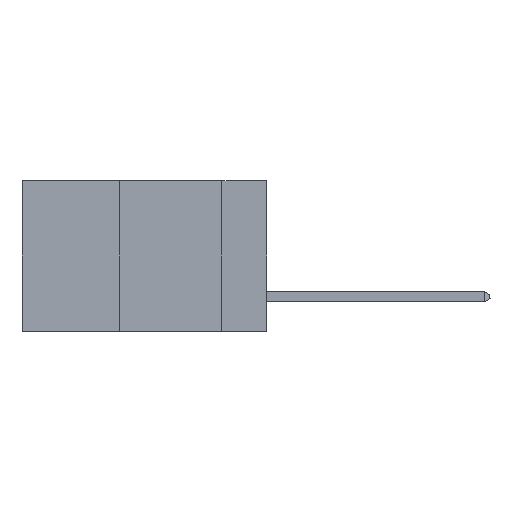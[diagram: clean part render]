
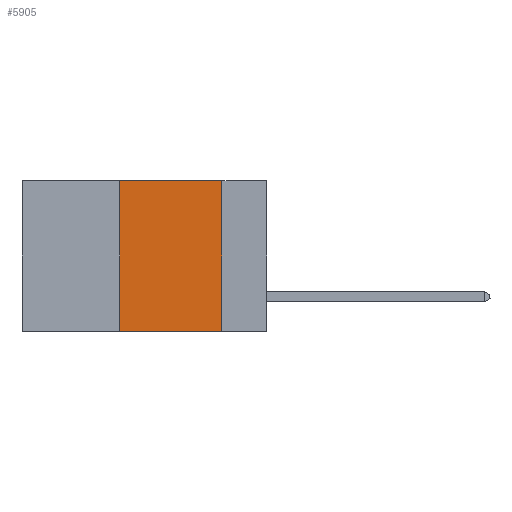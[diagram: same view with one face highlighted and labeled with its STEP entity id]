
A CAD part, left-side view. The second image highlights one B-rep face of the part: STEP entity #5905.
In plain terms, the highlighted planar face has unit normal (-1, 0, 0).
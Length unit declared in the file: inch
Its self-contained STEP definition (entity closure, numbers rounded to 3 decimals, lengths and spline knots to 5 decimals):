
#2057 = DIRECTION ( 'NONE',  ( 0., 0., -1. ) ) ;
#2290 = CARTESIAN_POINT ( 'NONE',  ( 0., 0.36, 0. ) ) ;
#3168 = DIRECTION ( 'NONE',  ( 0., 0., -1. ) ) ;
#3203 = VECTOR ( 'NONE', #41339, 39.37008 ) ;
#4285 = ORIENTED_EDGE ( 'NONE', *, *, #36678, .T. ) ;
#5442 = VERTEX_POINT ( 'NONE', #39004 ) ;
#5522 = LINE ( 'NONE', #34456, #35684 ) ;
#5905 = ADVANCED_FACE ( 'NONE', ( #32025 ), #12707, .F. ) ;
#6354 = LINE ( 'NONE', #30310, #41533 ) ;
#6455 = ORIENTED_EDGE ( 'NONE', *, *, #17333, .F. ) ;
#11524 = LINE ( 'NONE', #25259, #29942 ) ;
#12090 = DIRECTION ( 'NONE',  ( 0., 0., 1. ) ) ;
#12243 = EDGE_LOOP ( 'NONE', ( #38064, #12411, #6455, #4285 ) ) ;
#12411 = ORIENTED_EDGE ( 'NONE', *, *, #16439, .F. ) ;
#12707 = PLANE ( 'NONE',  #27489 ) ;
#15967 = DIRECTION ( 'NONE',  ( 0., -1., 0. ) ) ;
#16439 = EDGE_CURVE ( 'NONE', #20445, #27899, #11524, .T. ) ;
#17333 = EDGE_CURVE ( 'NONE', #5442, #20445, #6354, .T. ) ;
#20445 = VERTEX_POINT ( 'NONE', #2290 ) ;
#25259 = CARTESIAN_POINT ( 'NONE',  ( 0., 0.6, 0. ) ) ;
#25865 = CARTESIAN_POINT ( 'NONE',  ( 0., 0.6, 0. ) ) ;
#27489 = AXIS2_PLACEMENT_3D ( 'NONE', #25865, #42222, #3168 ) ;
#27899 = VERTEX_POINT ( 'NONE', #33735 ) ;
#28251 = CARTESIAN_POINT ( 'NONE',  ( 0., 0.6, -0.37 ) ) ;
#29942 = VECTOR ( 'NONE', #15967, 39.37008 ) ;
#30310 = CARTESIAN_POINT ( 'NONE',  ( 0., 0.36, 0. ) ) ;
#32025 = FACE_OUTER_BOUND ( 'NONE', #12243, .T. ) ;
#32193 = VERTEX_POINT ( 'NONE', #33381 ) ;
#33069 = EDGE_CURVE ( 'NONE', #27899, #32193, #5522, .T. ) ;
#33381 = CARTESIAN_POINT ( 'NONE',  ( 0., 0.11, -0.37 ) ) ;
#33735 = CARTESIAN_POINT ( 'NONE',  ( 0., 0.11, 0. ) ) ;
#34456 = CARTESIAN_POINT ( 'NONE',  ( 0., 0.11, 0. ) ) ;
#35684 = VECTOR ( 'NONE', #2057, 39.37008 ) ;
#36678 = EDGE_CURVE ( 'NONE', #5442, #32193, #37927, .T. ) ;
#37927 = LINE ( 'NONE', #28251, #3203 ) ;
#38064 = ORIENTED_EDGE ( 'NONE', *, *, #33069, .F. ) ;
#39004 = CARTESIAN_POINT ( 'NONE',  ( 0., 0.36, -0.37 ) ) ;
#41339 = DIRECTION ( 'NONE',  ( 0., -1., 0. ) ) ;
#41533 = VECTOR ( 'NONE', #12090, 39.37008 ) ;
#42222 = DIRECTION ( 'NONE',  ( 1., 0., 0. ) ) ;
